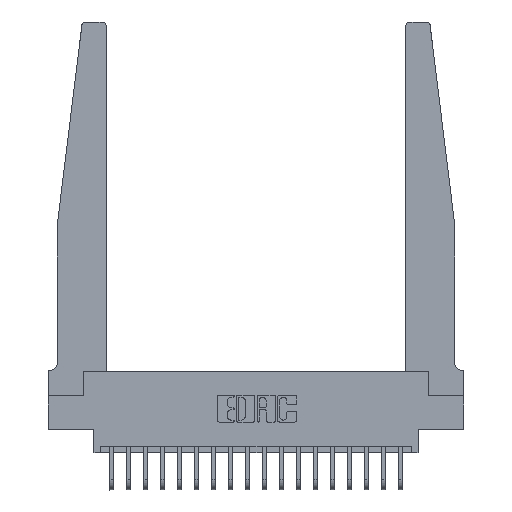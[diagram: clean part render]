
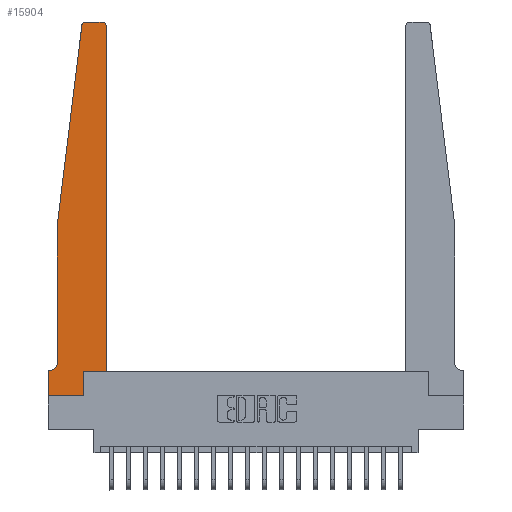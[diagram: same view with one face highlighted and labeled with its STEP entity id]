
A CAD part, top view. The second image highlights one B-rep face of the part: STEP entity #15904.
In plain terms, the highlighted planar face has unit normal (0, 0, 1).
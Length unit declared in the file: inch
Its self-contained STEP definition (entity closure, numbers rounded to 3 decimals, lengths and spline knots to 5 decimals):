
#351 = VERTEX_POINT ( 'NONE', #10979 ) ;
#544 = DIRECTION ( 'NONE',  ( 0., 0., 1. ) ) ;
#599 = ORIENTED_EDGE ( 'NONE', *, *, #15584, .T. ) ;
#705 = DIRECTION ( 'NONE',  ( 0., -1., 0. ) ) ;
#843 = FACE_OUTER_BOUND ( 'NONE', #17340, .T. ) ;
#847 = AXIS2_PLACEMENT_3D ( 'NONE', #12299, #18423, #10805 ) ;
#884 = CARTESIAN_POINT ( 'NONE',  ( 0.425, 0.18, 0.37 ) ) ;
#1201 = ORIENTED_EDGE ( 'NONE', *, *, #7012, .T. ) ;
#2022 = VECTOR ( 'NONE', #705, 39.37008 ) ;
#2054 = PLANE ( 'NONE',  #16236 ) ;
#2078 = ORIENTED_EDGE ( 'NONE', *, *, #9649, .T. ) ;
#2192 = CARTESIAN_POINT ( 'NONE',  ( 0.065, 0.1875, 0.37 ) ) ;
#2357 = CARTESIAN_POINT ( 'NONE',  ( 0., 0.1875, 0.37 ) ) ;
#2759 = ORIENTED_EDGE ( 'NONE', *, *, #6479, .T. ) ;
#2993 = CIRCLE ( 'NONE', #3622, 0.03 ) ;
#3091 = ORIENTED_EDGE ( 'NONE', *, *, #13603, .T. ) ;
#3344 = VERTEX_POINT ( 'NONE', #6929 ) ;
#3622 = AXIS2_PLACEMENT_3D ( 'NONE', #16014, #5466, #8574 ) ;
#4102 = CARTESIAN_POINT ( 'NONE',  ( 0.425, 0.18, 0.37 ) ) ;
#4260 = EDGE_CURVE ( 'NONE', #351, #14051, #8250, .T. ) ;
#4290 = CARTESIAN_POINT ( 'NONE',  ( 0.425, 2.72, 0.37 ) ) ;
#4893 = VECTOR ( 'NONE', #14912, 39.37008 ) ;
#4991 = DIRECTION ( 'NONE',  ( -1., 0., 0. ) ) ;
#5103 = DIRECTION ( 'NONE',  ( -1., 0., 0. ) ) ;
#5121 = VECTOR ( 'NONE', #8603, 39.37008 ) ;
#5466 = DIRECTION ( 'NONE',  ( 0., 0., 1. ) ) ;
#5599 = VECTOR ( 'NONE', #9956, 39.37008 ) ;
#5606 = CARTESIAN_POINT ( 'NONE',  ( 0.015, 0.2375, 0.37 ) ) ;
#6479 = EDGE_CURVE ( 'NONE', #14051, #15299, #19330, .T. ) ;
#6548 = DIRECTION ( 'NONE',  ( 1., 0., 0. ) ) ;
#6929 = CARTESIAN_POINT ( 'NONE',  ( 0., 0., 0.37 ) ) ;
#7012 = EDGE_CURVE ( 'NONE', #15779, #351, #9985, .T. ) ;
#7041 = LINE ( 'NONE', #9663, #5599 ) ;
#7123 = EDGE_CURVE ( 'NONE', #3344, #15779, #16595, .T. ) ;
#7267 = VERTEX_POINT ( 'NONE', #9361 ) ;
#7694 = EDGE_CURVE ( 'NONE', #10660, #9891, #12727, .T. ) ;
#8250 = LINE ( 'NONE', #12870, #13715 ) ;
#8477 = CARTESIAN_POINT ( 'NONE',  ( 0.2605, 0.18, 0.37 ) ) ;
#8574 = DIRECTION ( 'NONE',  ( 1., 0., 0. ) ) ;
#8603 = DIRECTION ( 'NONE',  ( 0., 1., 0. ) ) ;
#8618 = DIRECTION ( 'NONE',  ( -1., 0., 0. ) ) ;
#8868 = CARTESIAN_POINT ( 'NONE',  ( 0.2605, 0., 0.37 ) ) ;
#9151 = CARTESIAN_POINT ( 'NONE',  ( 0., 0.1875, 0.37 ) ) ;
#9169 = VERTEX_POINT ( 'NONE', #9151 ) ;
#9361 = CARTESIAN_POINT ( 'NONE',  ( 0.065, 0.2375, 0.37 ) ) ;
#9589 = CARTESIAN_POINT ( 'NONE',  ( 0.065, 1.25, 0.37 ) ) ;
#9638 = VECTOR ( 'NONE', #14606, 39.37008 ) ;
#9649 = EDGE_CURVE ( 'NONE', #9169, #3344, #14254, .T. ) ;
#9663 = CARTESIAN_POINT ( 'NONE',  ( 0.065, 1.25, 0.37 ) ) ;
#9799 = EDGE_CURVE ( 'NONE', #7267, #16498, #18355, .T. ) ;
#9891 = VERTEX_POINT ( 'NONE', #15226 ) ;
#9904 = LINE ( 'NONE', #2192, #19020 ) ;
#9956 = DIRECTION ( 'NONE',  ( -0.122, -0.992, 0. ) ) ;
#9985 = LINE ( 'NONE', #8477, #9638 ) ;
#10270 = CARTESIAN_POINT ( 'NONE',  ( 0.24675, 2.72367, 0.37 ) ) ;
#10310 = ORIENTED_EDGE ( 'NONE', *, *, #7694, .T. ) ;
#10660 = VERTEX_POINT ( 'NONE', #12890 ) ;
#10805 = DIRECTION ( 'NONE',  ( 1., 0., 0. ) ) ;
#10979 = CARTESIAN_POINT ( 'NONE',  ( 0.2605, 0.18, 0.37 ) ) ;
#11261 = EDGE_CURVE ( 'NONE', #16498, #9169, #9904, .T. ) ;
#11327 = EDGE_CURVE ( 'NONE', #19286, #7267, #15939, .T. ) ;
#11477 = DIRECTION ( 'NONE',  ( 1., 0., 0. ) ) ;
#11685 = EDGE_CURVE ( 'NONE', #9891, #12188, #2993, .T. ) ;
#12188 = VERTEX_POINT ( 'NONE', #10270 ) ;
#12299 = CARTESIAN_POINT ( 'NONE',  ( 0.395, 2.72, 0.37 ) ) ;
#12727 = LINE ( 'NONE', #18849, #13187 ) ;
#12846 = CARTESIAN_POINT ( 'NONE',  ( 0., 0., 0.37 ) ) ;
#12870 = CARTESIAN_POINT ( 'NONE',  ( 0.425, 0.18, 0.37 ) ) ;
#12890 = CARTESIAN_POINT ( 'NONE',  ( 0.395, 2.75, 0.37 ) ) ;
#12909 = AXIS2_PLACEMENT_3D ( 'NONE', #5606, #14840, #8618 ) ;
#13187 = VECTOR ( 'NONE', #5103, 39.37008 ) ;
#13284 = ORIENTED_EDGE ( 'NONE', *, *, #7123, .T. ) ;
#13385 = CARTESIAN_POINT ( 'NONE',  ( 0., 0., 0.37 ) ) ;
#13603 = EDGE_CURVE ( 'NONE', #12188, #19286, #7041, .T. ) ;
#13715 = VECTOR ( 'NONE', #6548, 39.37008 ) ;
#14020 = CARTESIAN_POINT ( 'NONE',  ( 0.015, 0.1875, 0.37 ) ) ;
#14051 = VERTEX_POINT ( 'NONE', #4102 ) ;
#14238 = ORIENTED_EDGE ( 'NONE', *, *, #11327, .T. ) ;
#14254 = LINE ( 'NONE', #12846, #2022 ) ;
#14309 = CIRCLE ( 'NONE', #847, 0.03 ) ;
#14606 = DIRECTION ( 'NONE',  ( 0., 1., 0. ) ) ;
#14840 = DIRECTION ( 'NONE',  ( 0., 0., -1. ) ) ;
#14900 = ORIENTED_EDGE ( 'NONE', *, *, #11261, .T. ) ;
#14912 = DIRECTION ( 'NONE',  ( 0., -1., 0. ) ) ;
#15226 = CARTESIAN_POINT ( 'NONE',  ( 0.27653, 2.75, 0.37 ) ) ;
#15299 = VERTEX_POINT ( 'NONE', #4290 ) ;
#15584 = EDGE_CURVE ( 'NONE', #15299, #10660, #14309, .T. ) ;
#15743 = VECTOR ( 'NONE', #19505, 39.37008 ) ;
#15779 = VERTEX_POINT ( 'NONE', #8868 ) ;
#15904 = ADVANCED_FACE ( 'NONE', ( #843 ), #2054, .T. ) ;
#15939 = LINE ( 'NONE', #16515, #4893 ) ;
#16014 = CARTESIAN_POINT ( 'NONE',  ( 0.27653, 2.72, 0.37 ) ) ;
#16236 = AXIS2_PLACEMENT_3D ( 'NONE', #2357, #544, #11477 ) ;
#16454 = ORIENTED_EDGE ( 'NONE', *, *, #9799, .T. ) ;
#16498 = VERTEX_POINT ( 'NONE', #14020 ) ;
#16515 = CARTESIAN_POINT ( 'NONE',  ( 0.065, 1.25, 0.37 ) ) ;
#16595 = LINE ( 'NONE', #13385, #15743 ) ;
#17340 = EDGE_LOOP ( 'NONE', ( #10310, #18019, #3091, #14238, #16454, #14900, #2078, #13284, #1201, #18021, #2759, #599 ) ) ;
#18019 = ORIENTED_EDGE ( 'NONE', *, *, #11685, .T. ) ;
#18021 = ORIENTED_EDGE ( 'NONE', *, *, #4260, .T. ) ;
#18355 = CIRCLE ( 'NONE', #12909, 0.05 ) ;
#18423 = DIRECTION ( 'NONE',  ( 0., 0., 1. ) ) ;
#18849 = CARTESIAN_POINT ( 'NONE',  ( 0.25, 2.75, 0.37 ) ) ;
#19020 = VECTOR ( 'NONE', #4991, 39.37008 ) ;
#19286 = VERTEX_POINT ( 'NONE', #9589 ) ;
#19330 = LINE ( 'NONE', #884, #5121 ) ;
#19505 = DIRECTION ( 'NONE',  ( 1., 0., 0. ) ) ;
